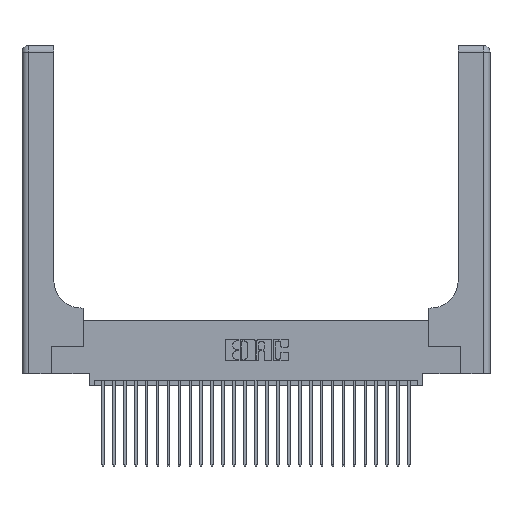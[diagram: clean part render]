
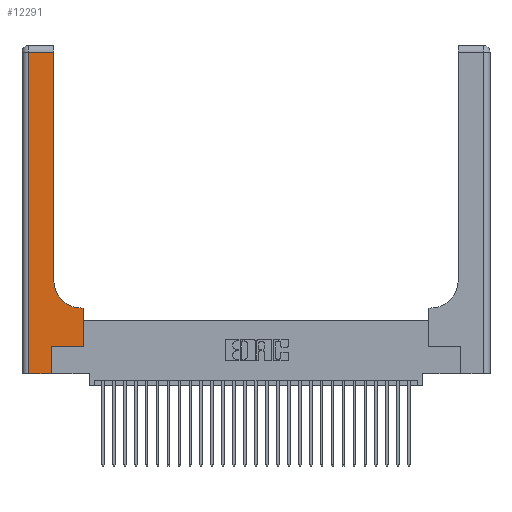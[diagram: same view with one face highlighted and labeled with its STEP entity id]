
A CAD part, top view. The second image highlights one B-rep face of the part: STEP entity #12291.
In plain terms, the highlighted planar face has unit normal (0, 0, 1).
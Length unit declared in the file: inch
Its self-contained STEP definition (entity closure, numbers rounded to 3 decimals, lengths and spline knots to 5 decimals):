
#223 = DIRECTION ( 'NONE',  ( 1., 0., 0. ) ) ;
#363 = VECTOR ( 'NONE', #19756, 39.37008 ) ;
#567 = CARTESIAN_POINT ( 'NONE',  ( 0.269, 0.25, 0.37 ) ) ;
#722 = AXIS2_PLACEMENT_3D ( 'NONE', #11814, #27783, #14123 ) ;
#783 = CARTESIAN_POINT ( 'NONE',  ( 0., 3., 0.37 ) ) ;
#908 = EDGE_CURVE ( 'NONE', #9180, #21173, #7024, .T. ) ;
#2851 = VERTEX_POINT ( 'NONE', #14240 ) ;
#3538 = AXIS2_PLACEMENT_3D ( 'NONE', #783, #5551, #21656 ) ;
#3547 = CARTESIAN_POINT ( 'NONE',  ( 0.06, 3., 0.37 ) ) ;
#3667 = CARTESIAN_POINT ( 'NONE',  ( 0.2915, 0.6, 0.37 ) ) ;
#3978 = VERTEX_POINT ( 'NONE', #7031 ) ;
#4309 = LINE ( 'NONE', #21105, #28018 ) ;
#4410 = VERTEX_POINT ( 'NONE', #24348 ) ;
#4460 = EDGE_LOOP ( 'NONE', ( #25523, #26944, #9426, #28376, #10867, #29066, #18428, #6904, #8346 ) ) ;
#4580 = LINE ( 'NONE', #3547, #22256 ) ;
#4980 = VERTEX_POINT ( 'NONE', #18650 ) ;
#5551 = DIRECTION ( 'NONE',  ( 0., 0., -1. ) ) ;
#5577 = CARTESIAN_POINT ( 'NONE',  ( 0., 0., 0.37 ) ) ;
#5640 = LINE ( 'NONE', #5577, #16503 ) ;
#5806 = CARTESIAN_POINT ( 'NONE',  ( 0.5585, 0.25, 0.37 ) ) ;
#5936 = DIRECTION ( 'NONE',  ( 0., -1., 0. ) ) ;
#6454 = CARTESIAN_POINT ( 'NONE',  ( 0.269, 0., 0.37 ) ) ;
#6904 = ORIENTED_EDGE ( 'NONE', *, *, #20560, .T. ) ;
#7024 = LINE ( 'NONE', #567, #24586 ) ;
#7031 = CARTESIAN_POINT ( 'NONE',  ( 0.269, 0., 0.37 ) ) ;
#7407 = LINE ( 'NONE', #3667, #363 ) ;
#7435 = EDGE_CURVE ( 'NONE', #17791, #2851, #22333, .T. ) ;
#7921 = DIRECTION ( 'NONE',  ( 1., 0., 0. ) ) ;
#8346 = ORIENTED_EDGE ( 'NONE', *, *, #10316, .T. ) ;
#8804 = EDGE_CURVE ( 'NONE', #2851, #18403, #4580, .T. ) ;
#9180 = VERTEX_POINT ( 'NONE', #13884 ) ;
#9360 = CARTESIAN_POINT ( 'NONE',  ( 0., 2.94, 0.37 ) ) ;
#9426 = ORIENTED_EDGE ( 'NONE', *, *, #8804, .T. ) ;
#10145 = VECTOR ( 'NONE', #25359, 39.37008 ) ;
#10316 = EDGE_CURVE ( 'NONE', #4410, #19441, #25343, .T. ) ;
#10555 = VECTOR ( 'NONE', #29640, 39.37008 ) ;
#10652 = VECTOR ( 'NONE', #22522, 39.37008 ) ;
#10867 = ORIENTED_EDGE ( 'NONE', *, *, #20666, .T. ) ;
#11814 = CARTESIAN_POINT ( 'NONE',  ( 0.5415, 0.85, 0.37 ) ) ;
#12291 = ADVANCED_FACE ( 'NONE', ( #18475 ), #28388, .F. ) ;
#13884 = CARTESIAN_POINT ( 'NONE',  ( 0.269, 0.25, 0.37 ) ) ;
#14123 = DIRECTION ( 'NONE',  ( 1., 0., 0. ) ) ;
#14240 = CARTESIAN_POINT ( 'NONE',  ( 0.06, 2.94, 0.37 ) ) ;
#16503 = VECTOR ( 'NONE', #7921, 39.37008 ) ;
#16616 = DIRECTION ( 'NONE',  ( 0., 1., 0. ) ) ;
#17791 = VERTEX_POINT ( 'NONE', #18680 ) ;
#18342 = EDGE_CURVE ( 'NONE', #21173, #4980, #22738, .T. ) ;
#18403 = VERTEX_POINT ( 'NONE', #23012 ) ;
#18428 = ORIENTED_EDGE ( 'NONE', *, *, #18342, .T. ) ;
#18475 = FACE_OUTER_BOUND ( 'NONE', #4460, .T. ) ;
#18650 = CARTESIAN_POINT ( 'NONE',  ( 0.5585, 0.6, 0.37 ) ) ;
#18680 = CARTESIAN_POINT ( 'NONE',  ( 0.2915, 2.94, 0.37 ) ) ;
#19441 = VERTEX_POINT ( 'NONE', #27023 ) ;
#19756 = DIRECTION ( 'NONE',  ( -1., 0., 0. ) ) ;
#20560 = EDGE_CURVE ( 'NONE', #4980, #4410, #7407, .T. ) ;
#20666 = EDGE_CURVE ( 'NONE', #3978, #9180, #22134, .T. ) ;
#21105 = CARTESIAN_POINT ( 'NONE',  ( 0.2915, 3., 0.37 ) ) ;
#21173 = VERTEX_POINT ( 'NONE', #5806 ) ;
#21656 = DIRECTION ( 'NONE',  ( -1., 0., 0. ) ) ;
#22134 = LINE ( 'NONE', #6454, #10652 ) ;
#22256 = VECTOR ( 'NONE', #5936, 39.37008 ) ;
#22333 = LINE ( 'NONE', #9360, #10145 ) ;
#22522 = DIRECTION ( 'NONE',  ( 0., 1., 0. ) ) ;
#22738 = LINE ( 'NONE', #29445, #10555 ) ;
#22866 = EDGE_CURVE ( 'NONE', #19441, #17791, #4309, .T. ) ;
#23012 = CARTESIAN_POINT ( 'NONE',  ( 0.06, 0., 0.37 ) ) ;
#24348 = CARTESIAN_POINT ( 'NONE',  ( 0.5415, 0.6, 0.37 ) ) ;
#24586 = VECTOR ( 'NONE', #223, 39.37008 ) ;
#25343 = CIRCLE ( 'NONE', #722, 0.25 ) ;
#25359 = DIRECTION ( 'NONE',  ( -1., 0., 0. ) ) ;
#25523 = ORIENTED_EDGE ( 'NONE', *, *, #22866, .T. ) ;
#26288 = EDGE_CURVE ( 'NONE', #18403, #3978, #5640, .T. ) ;
#26944 = ORIENTED_EDGE ( 'NONE', *, *, #7435, .T. ) ;
#27023 = CARTESIAN_POINT ( 'NONE',  ( 0.2915, 0.85, 0.37 ) ) ;
#27783 = DIRECTION ( 'NONE',  ( 0., 0., -1. ) ) ;
#28018 = VECTOR ( 'NONE', #16616, 39.37008 ) ;
#28376 = ORIENTED_EDGE ( 'NONE', *, *, #26288, .T. ) ;
#28388 = PLANE ( 'NONE',  #3538 ) ;
#29066 = ORIENTED_EDGE ( 'NONE', *, *, #908, .T. ) ;
#29445 = CARTESIAN_POINT ( 'NONE',  ( 0.5585, 0.25, 0.37 ) ) ;
#29640 = DIRECTION ( 'NONE',  ( 0., 1., 0. ) ) ;
